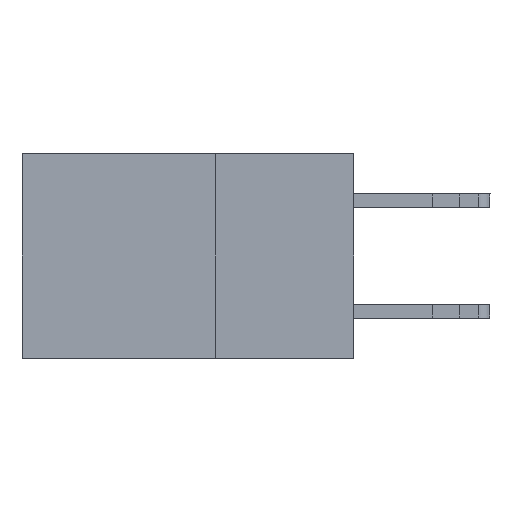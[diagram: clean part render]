
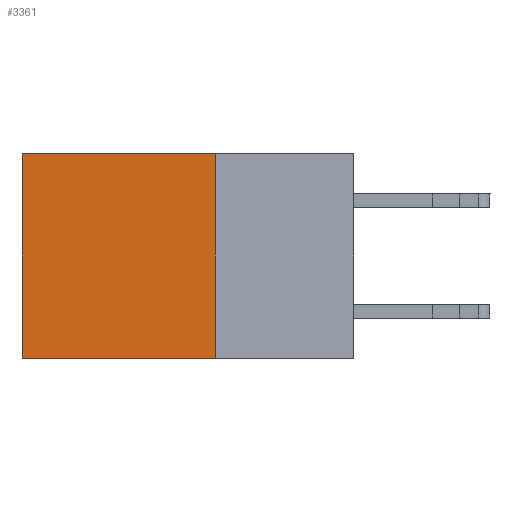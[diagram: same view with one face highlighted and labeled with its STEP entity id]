
A CAD part, left-side view. The second image highlights one B-rep face of the part: STEP entity #3361.
In plain terms, the highlighted planar face has unit normal (-1, 0, 0).
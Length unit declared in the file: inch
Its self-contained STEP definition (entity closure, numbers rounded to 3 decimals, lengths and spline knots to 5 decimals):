
#132 = ORIENTED_EDGE ( 'NONE', *, *, #9093, .T. ) ;
#295 = VERTEX_POINT ( 'NONE', #2027 ) ;
#410 = CARTESIAN_POINT ( 'NONE',  ( 0.2875, 0.25, 0. ) ) ;
#481 = VERTEX_POINT ( 'NONE', #17225 ) ;
#1500 = CARTESIAN_POINT ( 'NONE',  ( 0.2875, 0.6, 0. ) ) ;
#1591 = EDGE_CURVE ( 'NONE', #481, #10398, #6598, .T. ) ;
#1803 = DIRECTION ( 'NONE',  ( 0., 1., 0. ) ) ;
#2027 = CARTESIAN_POINT ( 'NONE',  ( 0.2875, 0.6, -0.37 ) ) ;
#2163 = DIRECTION ( 'NONE',  ( 1., 0., 0. ) ) ;
#2929 = LINE ( 'NONE', #410, #14074 ) ;
#3361 = ADVANCED_FACE ( 'NONE', ( #3528 ), #9477, .F. ) ;
#3528 = FACE_OUTER_BOUND ( 'NONE', #15629, .T. ) ;
#4377 = ORIENTED_EDGE ( 'NONE', *, *, #5645, .F. ) ;
#4957 = CARTESIAN_POINT ( 'NONE',  ( 0.2875, 0.25, 0. ) ) ;
#5066 = EDGE_CURVE ( 'NONE', #481, #9898, #2929, .T. ) ;
#5645 = EDGE_CURVE ( 'NONE', #9898, #295, #15094, .T. ) ;
#5903 = AXIS2_PLACEMENT_3D ( 'NONE', #4957, #2163, #15363 ) ;
#6598 = LINE ( 'NONE', #8400, #18956 ) ;
#8400 = CARTESIAN_POINT ( 'NONE',  ( 0.2875, 0.25, 0. ) ) ;
#8417 = CARTESIAN_POINT ( 'NONE',  ( 0.2875, 0.25, -0.37 ) ) ;
#8959 = CARTESIAN_POINT ( 'NONE',  ( 0.2875, 0.6, 0. ) ) ;
#9093 = EDGE_CURVE ( 'NONE', #10398, #295, #10178, .T. ) ;
#9177 = VECTOR ( 'NONE', #1803, 39.37008 ) ;
#9477 = PLANE ( 'NONE',  #5903 ) ;
#9898 = VERTEX_POINT ( 'NONE', #8417 ) ;
#10178 = LINE ( 'NONE', #1500, #17825 ) ;
#10398 = VERTEX_POINT ( 'NONE', #8959 ) ;
#13123 = ORIENTED_EDGE ( 'NONE', *, *, #5066, .F. ) ;
#13171 = DIRECTION ( 'NONE',  ( 0., 0., -1. ) ) ;
#13944 = CARTESIAN_POINT ( 'NONE',  ( 0.2875, 0.25, -0.37 ) ) ;
#14074 = VECTOR ( 'NONE', #17558, 39.37008 ) ;
#15094 = LINE ( 'NONE', #13944, #9177 ) ;
#15363 = DIRECTION ( 'NONE',  ( 0., 0., -1. ) ) ;
#15555 = DIRECTION ( 'NONE',  ( 0., 1., 0. ) ) ;
#15629 = EDGE_LOOP ( 'NONE', ( #132, #4377, #13123, #17125 ) ) ;
#17125 = ORIENTED_EDGE ( 'NONE', *, *, #1591, .T. ) ;
#17225 = CARTESIAN_POINT ( 'NONE',  ( 0.2875, 0.25, 0. ) ) ;
#17558 = DIRECTION ( 'NONE',  ( 0., 0., -1. ) ) ;
#17825 = VECTOR ( 'NONE', #13171, 39.37008 ) ;
#18956 = VECTOR ( 'NONE', #15555, 39.37008 ) ;
